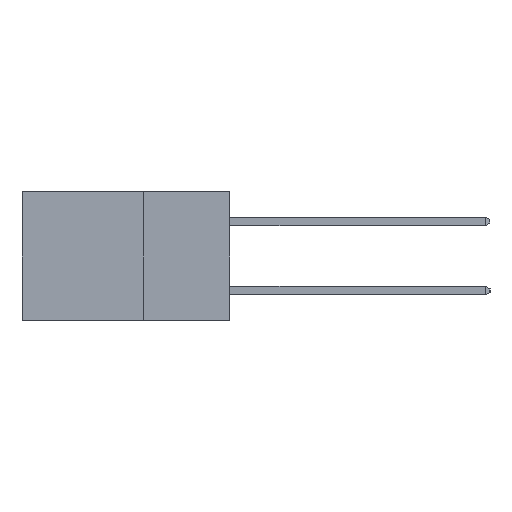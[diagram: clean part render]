
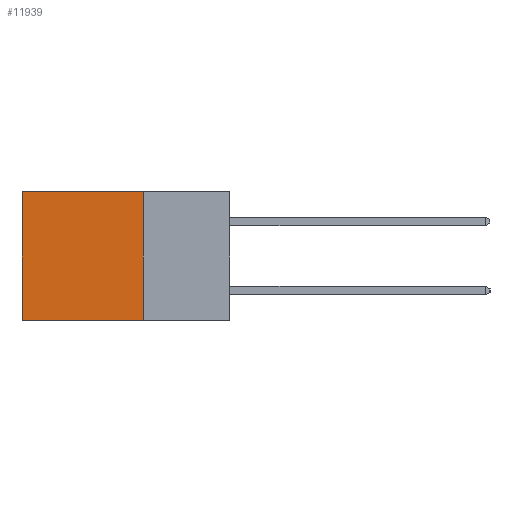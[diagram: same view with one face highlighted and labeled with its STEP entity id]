
A CAD part, left-side view. The second image highlights one B-rep face of the part: STEP entity #11939.
In plain terms, the highlighted planar face has unit normal (-1, 0, 0).
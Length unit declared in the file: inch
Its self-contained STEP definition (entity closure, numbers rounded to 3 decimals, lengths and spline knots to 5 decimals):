
#215 = LINE ( 'NONE', #1073, #5246 ) ;
#1011 = EDGE_CURVE ( 'NONE', #3787, #7615, #12737, .T. ) ;
#1040 = DIRECTION ( 'NONE',  ( 0., 0., -1. ) ) ;
#1073 = CARTESIAN_POINT ( 'NONE',  ( 0.2615, 0.6, -0.37 ) ) ;
#1197 = VERTEX_POINT ( 'NONE', #6586 ) ;
#1441 = LINE ( 'NONE', #7474, #3803 ) ;
#2209 = VECTOR ( 'NONE', #9534, 39.37008 ) ;
#2519 = EDGE_CURVE ( 'NONE', #1197, #3787, #7720, .T. ) ;
#3555 = CARTESIAN_POINT ( 'NONE',  ( 0.2615, 0.6, 0. ) ) ;
#3573 = ORIENTED_EDGE ( 'NONE', *, *, #2519, .F. ) ;
#3649 = FACE_OUTER_BOUND ( 'NONE', #11070, .T. ) ;
#3787 = VERTEX_POINT ( 'NONE', #11380 ) ;
#3803 = VECTOR ( 'NONE', #7489, 39.37008 ) ;
#4941 = DIRECTION ( 'NONE',  ( 0., 0., -1. ) ) ;
#4959 = DIRECTION ( 'NONE',  ( 1., 0., 0. ) ) ;
#4975 = CARTESIAN_POINT ( 'NONE',  ( 0.2615, 0.25, -0.37 ) ) ;
#4985 = PLANE ( 'NONE',  #10127 ) ;
#5246 = VECTOR ( 'NONE', #1040, 39.37008 ) ;
#6586 = CARTESIAN_POINT ( 'NONE',  ( 0.2615, 0.25, 0. ) ) ;
#6934 = ORIENTED_EDGE ( 'NONE', *, *, #11509, .T. ) ;
#7115 = ORIENTED_EDGE ( 'NONE', *, *, #1011, .F. ) ;
#7474 = CARTESIAN_POINT ( 'NONE',  ( 0.2615, 0.25, 0. ) ) ;
#7489 = DIRECTION ( 'NONE',  ( 0., 1., 0. ) ) ;
#7615 = VERTEX_POINT ( 'NONE', #10074 ) ;
#7720 = LINE ( 'NONE', #9486, #2209 ) ;
#9486 = CARTESIAN_POINT ( 'NONE',  ( 0.2615, 0.25, -0.37 ) ) ;
#9534 = DIRECTION ( 'NONE',  ( 0., 0., -1. ) ) ;
#9849 = VECTOR ( 'NONE', #11961, 39.37008 ) ;
#10074 = CARTESIAN_POINT ( 'NONE',  ( 0.2615, 0.6, -0.37 ) ) ;
#10127 = AXIS2_PLACEMENT_3D ( 'NONE', #4975, #4959, #4941 ) ;
#11070 = EDGE_LOOP ( 'NONE', ( #12179, #7115, #3573, #6934 ) ) ;
#11380 = CARTESIAN_POINT ( 'NONE',  ( 0.2615, 0.25, -0.37 ) ) ;
#11509 = EDGE_CURVE ( 'NONE', #1197, #12271, #1441, .T. ) ;
#11939 = ADVANCED_FACE ( 'NONE', ( #3649 ), #4985, .F. ) ;
#11961 = DIRECTION ( 'NONE',  ( 0., 1., 0. ) ) ;
#12179 = ORIENTED_EDGE ( 'NONE', *, *, #12802, .T. ) ;
#12271 = VERTEX_POINT ( 'NONE', #3555 ) ;
#12295 = CARTESIAN_POINT ( 'NONE',  ( 0.2615, 0.25, -0.37 ) ) ;
#12737 = LINE ( 'NONE', #12295, #9849 ) ;
#12802 = EDGE_CURVE ( 'NONE', #12271, #7615, #215, .T. ) ;
